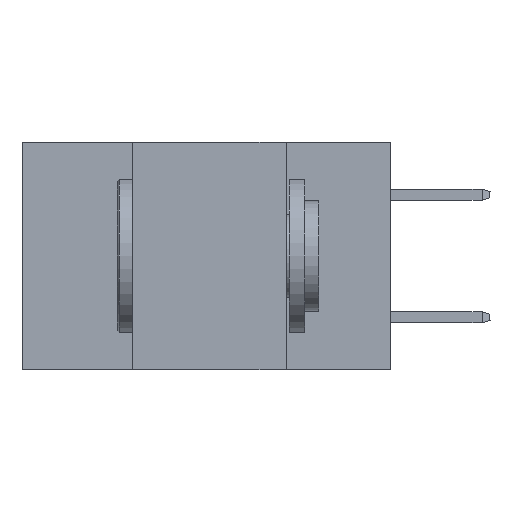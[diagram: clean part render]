
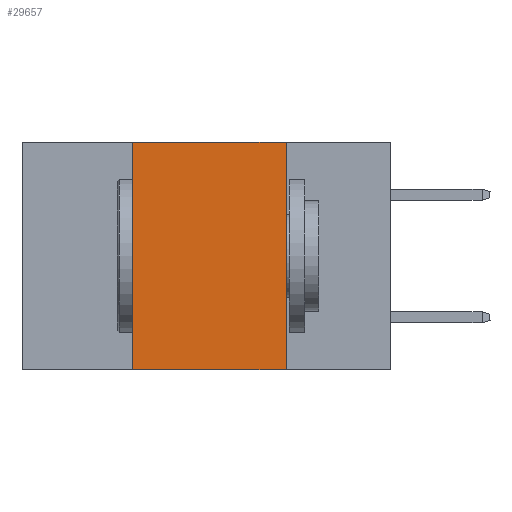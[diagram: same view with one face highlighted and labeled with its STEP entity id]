
A CAD part, left-side view. The second image highlights one B-rep face of the part: STEP entity #29657.
In plain terms, the highlighted planar face has unit normal (-1, 0, 0).
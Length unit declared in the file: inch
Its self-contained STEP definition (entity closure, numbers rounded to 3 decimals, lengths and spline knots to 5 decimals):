
#441 = LINE ( 'NONE', #6953, #33532 ) ;
#2629 = VERTEX_POINT ( 'NONE', #27224 ) ;
#2958 = ORIENTED_EDGE ( 'NONE', *, *, #21804, .F. ) ;
#3720 = FACE_OUTER_BOUND ( 'NONE', #4506, .T. ) ;
#4186 = DIRECTION ( 'NONE',  ( 0., 0., 1. ) ) ;
#4273 = DIRECTION ( 'NONE',  ( 1., 0., 0. ) ) ;
#4506 = EDGE_LOOP ( 'NONE', ( #2958, #16430, #21356, #28550 ) ) ;
#6953 = CARTESIAN_POINT ( 'NONE',  ( 0., 0.42, 0. ) ) ;
#8909 = EDGE_CURVE ( 'NONE', #30082, #2629, #31255, .T. ) ;
#9979 = VERTEX_POINT ( 'NONE', #26871 ) ;
#12983 = CARTESIAN_POINT ( 'NONE',  ( 0., 0.17, 0. ) ) ;
#14904 = EDGE_CURVE ( 'NONE', #16140, #9979, #31177, .T. ) ;
#16140 = VERTEX_POINT ( 'NONE', #33901 ) ;
#16156 = PLANE ( 'NONE',  #21888 ) ;
#16430 = ORIENTED_EDGE ( 'NONE', *, *, #14904, .F. ) ;
#17978 = VECTOR ( 'NONE', #18822, 39.37008 ) ;
#18822 = DIRECTION ( 'NONE',  ( 0., 0., -1. ) ) ;
#19731 = DIRECTION ( 'NONE',  ( 0., 0., -1. ) ) ;
#21356 = ORIENTED_EDGE ( 'NONE', *, *, #38873, .F. ) ;
#21804 = EDGE_CURVE ( 'NONE', #9979, #2629, #24601, .T. ) ;
#21888 = AXIS2_PLACEMENT_3D ( 'NONE', #34273, #4273, #19731 ) ;
#23195 = VECTOR ( 'NONE', #24762, 39.37008 ) ;
#24601 = LINE ( 'NONE', #12983, #17978 ) ;
#24762 = DIRECTION ( 'NONE',  ( 0., -1., 0. ) ) ;
#26871 = CARTESIAN_POINT ( 'NONE',  ( 0., 0.17, 0. ) ) ;
#27224 = CARTESIAN_POINT ( 'NONE',  ( 0., 0.17, -0.37 ) ) ;
#27389 = VECTOR ( 'NONE', #36624, 39.37008 ) ;
#28020 = CARTESIAN_POINT ( 'NONE',  ( 0., 0.42, -0.37 ) ) ;
#28550 = ORIENTED_EDGE ( 'NONE', *, *, #8909, .T. ) ;
#29657 = ADVANCED_FACE ( 'NONE', ( #3720 ), #16156, .F. ) ;
#30082 = VERTEX_POINT ( 'NONE', #28020 ) ;
#31177 = LINE ( 'NONE', #36372, #27389 ) ;
#31255 = LINE ( 'NONE', #33527, #23195 ) ;
#33527 = CARTESIAN_POINT ( 'NONE',  ( 0., 0.6, -0.37 ) ) ;
#33532 = VECTOR ( 'NONE', #4186, 39.37008 ) ;
#33901 = CARTESIAN_POINT ( 'NONE',  ( 0., 0.42, 0. ) ) ;
#34273 = CARTESIAN_POINT ( 'NONE',  ( 0., 0.6, 0. ) ) ;
#36372 = CARTESIAN_POINT ( 'NONE',  ( 0., 0.6, 0. ) ) ;
#36624 = DIRECTION ( 'NONE',  ( 0., -1., 0. ) ) ;
#38873 = EDGE_CURVE ( 'NONE', #30082, #16140, #441, .T. ) ;
